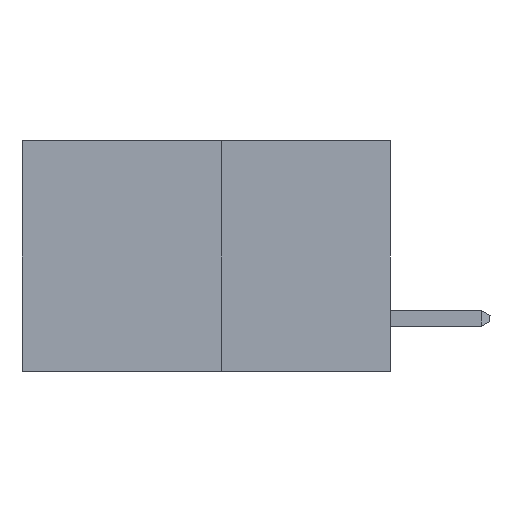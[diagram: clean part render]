
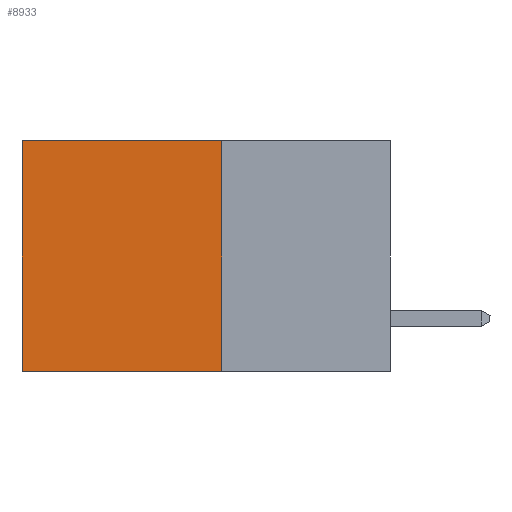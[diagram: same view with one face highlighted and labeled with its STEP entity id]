
A CAD part, left-side view. The second image highlights one B-rep face of the part: STEP entity #8933.
In plain terms, the highlighted planar face has unit normal (-1, 0, 0).
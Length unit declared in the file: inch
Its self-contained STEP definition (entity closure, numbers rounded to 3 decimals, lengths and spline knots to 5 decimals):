
#320 = VERTEX_POINT ( 'NONE', #18176 ) ;
#339 = ORIENTED_EDGE ( 'NONE', *, *, #6688, .F. ) ;
#449 = CARTESIAN_POINT ( 'NONE',  ( 0.277, 0.59, 0. ) ) ;
#1296 = ORIENTED_EDGE ( 'NONE', *, *, #6825, .F. ) ;
#1598 = EDGE_CURVE ( 'NONE', #12830, #320, #18977, .T. ) ;
#2437 = VERTEX_POINT ( 'NONE', #19028 ) ;
#2490 = FACE_OUTER_BOUND ( 'NONE', #14185, .T. ) ;
#2798 = VECTOR ( 'NONE', #12093, 39.37008 ) ;
#3106 = VECTOR ( 'NONE', #9047, 39.37008 ) ;
#4431 = VECTOR ( 'NONE', #18541, 39.37008 ) ;
#4567 = CARTESIAN_POINT ( 'NONE',  ( 0.277, 0.27, 0. ) ) ;
#5409 = LINE ( 'NONE', #18684, #4431 ) ;
#6642 = LINE ( 'NONE', #4567, #3106 ) ;
#6688 = EDGE_CURVE ( 'NONE', #8097, #320, #6804, .T. ) ;
#6804 = LINE ( 'NONE', #12928, #2798 ) ;
#6825 = EDGE_CURVE ( 'NONE', #2437, #8097, #5409, .T. ) ;
#6997 = VECTOR ( 'NONE', #12059, 39.37008 ) ;
#7390 = ORIENTED_EDGE ( 'NONE', *, *, #1598, .T. ) ;
#8097 = VERTEX_POINT ( 'NONE', #18693 ) ;
#8933 = ADVANCED_FACE ( 'NONE', ( #2490 ), #11406, .F. ) ;
#9047 = DIRECTION ( 'NONE',  ( 0., 1., 0. ) ) ;
#11325 = DIRECTION ( 'NONE',  ( 0., 0., -1. ) ) ;
#11341 = DIRECTION ( 'NONE',  ( 1., 0., 0. ) ) ;
#11363 = CARTESIAN_POINT ( 'NONE',  ( 0.277, 0.27, -0.37 ) ) ;
#11406 = PLANE ( 'NONE',  #18551 ) ;
#11977 = EDGE_CURVE ( 'NONE', #2437, #12830, #6642, .T. ) ;
#12059 = DIRECTION ( 'NONE',  ( 0., 0., -1. ) ) ;
#12093 = DIRECTION ( 'NONE',  ( 0., 1., 0. ) ) ;
#12830 = VERTEX_POINT ( 'NONE', #449 ) ;
#12928 = CARTESIAN_POINT ( 'NONE',  ( 0.277, 0.27, -0.37 ) ) ;
#13790 = ORIENTED_EDGE ( 'NONE', *, *, #11977, .T. ) ;
#14185 = EDGE_LOOP ( 'NONE', ( #7390, #339, #1296, #13790 ) ) ;
#14925 = CARTESIAN_POINT ( 'NONE',  ( 0.277, 0.59, -0.37 ) ) ;
#18176 = CARTESIAN_POINT ( 'NONE',  ( 0.277, 0.59, -0.37 ) ) ;
#18541 = DIRECTION ( 'NONE',  ( 0., 0., -1. ) ) ;
#18551 = AXIS2_PLACEMENT_3D ( 'NONE', #11363, #11341, #11325 ) ;
#18684 = CARTESIAN_POINT ( 'NONE',  ( 0.277, 0.27, -0.37 ) ) ;
#18693 = CARTESIAN_POINT ( 'NONE',  ( 0.277, 0.27, -0.37 ) ) ;
#18977 = LINE ( 'NONE', #14925, #6997 ) ;
#19028 = CARTESIAN_POINT ( 'NONE',  ( 0.277, 0.27, 0. ) ) ;
